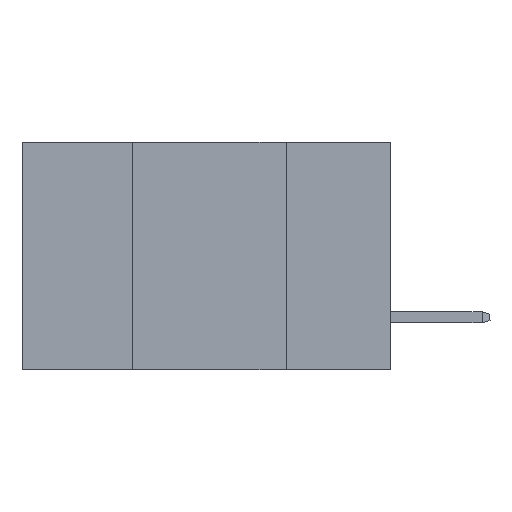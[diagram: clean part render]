
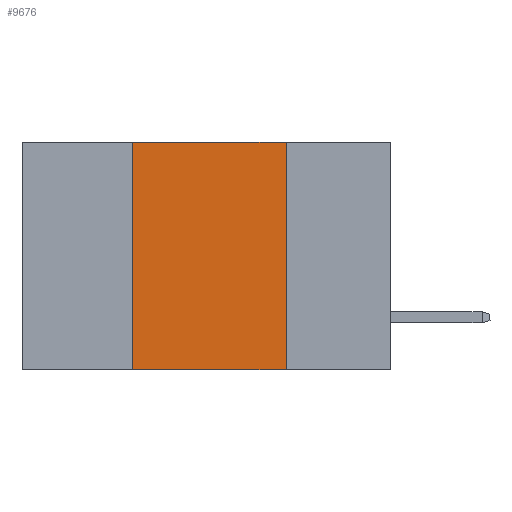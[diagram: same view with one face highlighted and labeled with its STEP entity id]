
A CAD part, left-side view. The second image highlights one B-rep face of the part: STEP entity #9676.
In plain terms, the highlighted planar face has unit normal (-1, 0, 0).
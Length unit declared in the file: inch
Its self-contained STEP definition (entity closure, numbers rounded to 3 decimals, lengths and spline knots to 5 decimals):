
#1186 = LINE ( 'NONE', #5350, #10432 ) ;
#2191 = AXIS2_PLACEMENT_3D ( 'NONE', #6763, #19540, #8594 ) ;
#2777 = VECTOR ( 'NONE', #5562, 39.37008 ) ;
#3248 = CARTESIAN_POINT ( 'NONE',  ( 0., 0.17, -0.37 ) ) ;
#3263 = ORIENTED_EDGE ( 'NONE', *, *, #22761, .F. ) ;
#3712 = CARTESIAN_POINT ( 'NONE',  ( 0., 0.42, 0. ) ) ;
#3838 = ORIENTED_EDGE ( 'NONE', *, *, #16927, .F. ) ;
#5066 = CARTESIAN_POINT ( 'NONE',  ( 0., 0.42, -0.37 ) ) ;
#5350 = CARTESIAN_POINT ( 'NONE',  ( 0., 0.17, 0. ) ) ;
#5562 = DIRECTION ( 'NONE',  ( 0., 0., 1. ) ) ;
#6387 = EDGE_CURVE ( 'NONE', #12243, #7860, #10735, .T. ) ;
#6763 = CARTESIAN_POINT ( 'NONE',  ( 0., 0.6, 0. ) ) ;
#7235 = DIRECTION ( 'NONE',  ( 0., 0., -1. ) ) ;
#7860 = VERTEX_POINT ( 'NONE', #3248 ) ;
#8299 = VERTEX_POINT ( 'NONE', #17511 ) ;
#8594 = DIRECTION ( 'NONE',  ( 0., 0., -1. ) ) ;
#9676 = ADVANCED_FACE ( 'NONE', ( #20953 ), #21270, .F. ) ;
#9772 = DIRECTION ( 'NONE',  ( 0., -1., 0. ) ) ;
#10432 = VECTOR ( 'NONE', #7235, 39.37008 ) ;
#10735 = LINE ( 'NONE', #15160, #15023 ) ;
#11521 = CARTESIAN_POINT ( 'NONE',  ( 0., 0.17, 0. ) ) ;
#12225 = LINE ( 'NONE', #18879, #16530 ) ;
#12243 = VERTEX_POINT ( 'NONE', #5066 ) ;
#12527 = LINE ( 'NONE', #3712, #2777 ) ;
#15023 = VECTOR ( 'NONE', #15233, 39.37008 ) ;
#15160 = CARTESIAN_POINT ( 'NONE',  ( 0., 0.6, -0.37 ) ) ;
#15233 = DIRECTION ( 'NONE',  ( 0., -1., 0. ) ) ;
#16530 = VECTOR ( 'NONE', #9772, 39.37008 ) ;
#16927 = EDGE_CURVE ( 'NONE', #8299, #19768, #12225, .T. ) ;
#17301 = ORIENTED_EDGE ( 'NONE', *, *, #20761, .F. ) ;
#17511 = CARTESIAN_POINT ( 'NONE',  ( 0., 0.42, 0. ) ) ;
#18879 = CARTESIAN_POINT ( 'NONE',  ( 0., 0.6, 0. ) ) ;
#19540 = DIRECTION ( 'NONE',  ( 1., 0., 0. ) ) ;
#19768 = VERTEX_POINT ( 'NONE', #11521 ) ;
#20761 = EDGE_CURVE ( 'NONE', #12243, #8299, #12527, .T. ) ;
#20953 = FACE_OUTER_BOUND ( 'NONE', #21679, .T. ) ;
#21270 = PLANE ( 'NONE',  #2191 ) ;
#21604 = ORIENTED_EDGE ( 'NONE', *, *, #6387, .T. ) ;
#21679 = EDGE_LOOP ( 'NONE', ( #3263, #3838, #17301, #21604 ) ) ;
#22761 = EDGE_CURVE ( 'NONE', #19768, #7860, #1186, .T. ) ;
